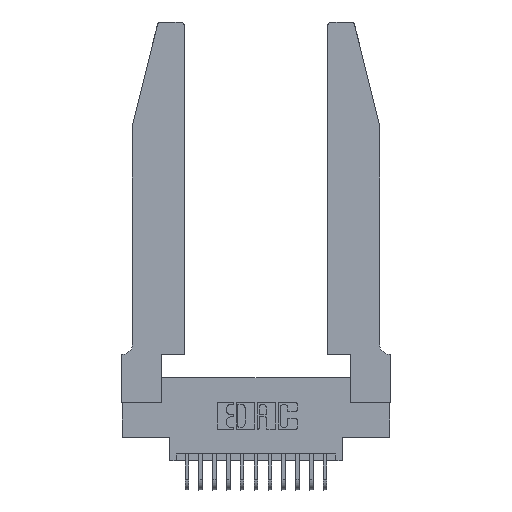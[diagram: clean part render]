
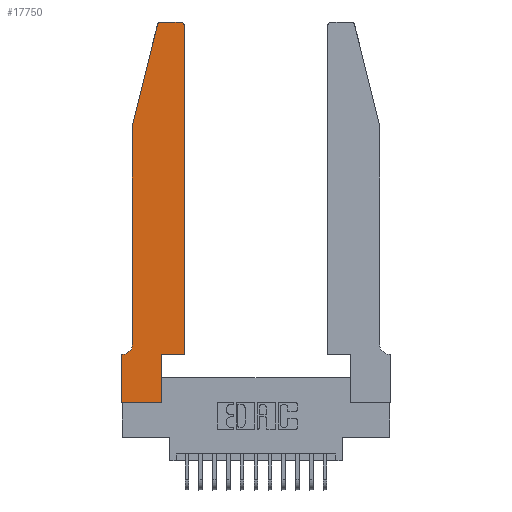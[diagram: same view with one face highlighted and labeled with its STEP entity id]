
A CAD part, top view. The second image highlights one B-rep face of the part: STEP entity #17750.
In plain terms, the highlighted planar face has unit normal (0, 0, 1).
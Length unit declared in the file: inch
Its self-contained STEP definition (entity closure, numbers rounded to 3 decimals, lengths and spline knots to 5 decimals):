
#214 = EDGE_CURVE ( 'NONE', #11306, #16267, #1139, .T. ) ;
#298 = DIRECTION ( 'NONE',  ( -1., 0., 0. ) ) ;
#438 = DIRECTION ( 'NONE',  ( 1., 0., 0. ) ) ;
#689 = AXIS2_PLACEMENT_3D ( 'NONE', #11157, #15512, #16883 ) ;
#804 = ORIENTED_EDGE ( 'NONE', *, *, #7151, .T. ) ;
#845 = ORIENTED_EDGE ( 'NONE', *, *, #3106, .T. ) ;
#929 = CARTESIAN_POINT ( 'NONE',  ( 0.4205, 2.72, 0.37 ) ) ;
#1097 = CARTESIAN_POINT ( 'NONE',  ( 0.0055, 0.35, 0.37 ) ) ;
#1134 = VECTOR ( 'NONE', #3983, 39.37008 ) ;
#1139 = LINE ( 'NONE', #12111, #13782 ) ;
#1180 = DIRECTION ( 'NONE',  ( 0., -1., 0. ) ) ;
#1259 = VERTEX_POINT ( 'NONE', #16466 ) ;
#1511 = VERTEX_POINT ( 'NONE', #18395 ) ;
#1604 = DIRECTION ( 'NONE',  ( 0., 1., 0. ) ) ;
#1765 = VERTEX_POINT ( 'NONE', #13237 ) ;
#1793 = DIRECTION ( 'NONE',  ( -1., 0., 0. ) ) ;
#1834 = EDGE_CURVE ( 'NONE', #12847, #3336, #16252, .T. ) ;
#2216 = LINE ( 'NONE', #17398, #12274 ) ;
#2345 = CARTESIAN_POINT ( 'NONE',  ( 0.0755, 0.35, 0.37 ) ) ;
#2641 = ORIENTED_EDGE ( 'NONE', *, *, #6393, .T. ) ;
#3106 = EDGE_CURVE ( 'NONE', #5735, #12847, #17629, .T. ) ;
#3282 = VERTEX_POINT ( 'NONE', #12560 ) ;
#3287 = VECTOR ( 'NONE', #438, 39.37008 ) ;
#3297 = CARTESIAN_POINT ( 'NONE',  ( 0.2865, 0., 0.37 ) ) ;
#3336 = VERTEX_POINT ( 'NONE', #1097 ) ;
#3373 = ORIENTED_EDGE ( 'NONE', *, *, #16294, .T. ) ;
#3421 = DIRECTION ( 'NONE',  ( 1., 0., 0. ) ) ;
#3604 = ORIENTED_EDGE ( 'NONE', *, *, #1834, .T. ) ;
#3788 = CARTESIAN_POINT ( 'NONE',  ( 0., 0., 0.37 ) ) ;
#3844 = VECTOR ( 'NONE', #7326, 39.37008 ) ;
#3961 = DIRECTION ( 'NONE',  ( 1., 0., 0. ) ) ;
#3983 = DIRECTION ( 'NONE',  ( -1., 0., 0. ) ) ;
#4712 = CARTESIAN_POINT ( 'NONE',  ( 0., 0.35, 0.37 ) ) ;
#5204 = AXIS2_PLACEMENT_3D ( 'NONE', #929, #5391, #3961 ) ;
#5363 = ORIENTED_EDGE ( 'NONE', *, *, #14407, .T. ) ;
#5391 = DIRECTION ( 'NONE',  ( 0., 0., 1. ) ) ;
#5583 = DIRECTION ( 'NONE',  ( -0.239, -0.971, 0. ) ) ;
#5711 = CARTESIAN_POINT ( 'NONE',  ( 0.0755, 0.42, 0.37 ) ) ;
#5735 = VERTEX_POINT ( 'NONE', #15242 ) ;
#6230 = PLANE ( 'NONE',  #6342 ) ;
#6342 = AXIS2_PLACEMENT_3D ( 'NONE', #4712, #7707, #3421 ) ;
#6393 = EDGE_CURVE ( 'NONE', #15076, #12180, #7017, .T. ) ;
#6853 = EDGE_CURVE ( 'NONE', #3282, #1259, #17033, .T. ) ;
#6996 = LINE ( 'NONE', #2345, #1134 ) ;
#7017 = LINE ( 'NONE', #12567, #3287 ) ;
#7028 = EDGE_CURVE ( 'NONE', #1259, #1511, #18914, .T. ) ;
#7151 = EDGE_CURVE ( 'NONE', #10709, #15076, #17489, .T. ) ;
#7326 = DIRECTION ( 'NONE',  ( 0., 1., 0. ) ) ;
#7532 = VECTOR ( 'NONE', #1604, 39.37008 ) ;
#7707 = DIRECTION ( 'NONE',  ( 0., 0., 1. ) ) ;
#9122 = CARTESIAN_POINT ( 'NONE',  ( 0.2865, 0.35, 0.37 ) ) ;
#9790 = VECTOR ( 'NONE', #17410, 39.37008 ) ;
#10137 = ORIENTED_EDGE ( 'NONE', *, *, #19091, .T. ) ;
#10580 = CARTESIAN_POINT ( 'NONE',  ( 0., 0., 0.37 ) ) ;
#10596 = LINE ( 'NONE', #19210, #3844 ) ;
#10644 = VECTOR ( 'NONE', #1180, 39.37008 ) ;
#10709 = VERTEX_POINT ( 'NONE', #11297 ) ;
#10827 = ORIENTED_EDGE ( 'NONE', *, *, #7028, .T. ) ;
#10984 = EDGE_CURVE ( 'NONE', #1511, #5735, #2216, .T. ) ;
#11157 = CARTESIAN_POINT ( 'NONE',  ( 0.284, 2.72, 0.37 ) ) ;
#11297 = CARTESIAN_POINT ( 'NONE',  ( 0., 0.35, 0.37 ) ) ;
#11306 = VERTEX_POINT ( 'NONE', #17693 ) ;
#11874 = CIRCLE ( 'NONE', #5204, 0.03 ) ;
#12111 = CARTESIAN_POINT ( 'NONE',  ( 0.4505, 0.35, 0.37 ) ) ;
#12179 = ORIENTED_EDGE ( 'NONE', *, *, #10984, .T. ) ;
#12180 = VERTEX_POINT ( 'NONE', #3297 ) ;
#12274 = VECTOR ( 'NONE', #5583, 39.37008 ) ;
#12286 = FACE_OUTER_BOUND ( 'NONE', #13163, .T. ) ;
#12386 = VECTOR ( 'NONE', #298, 39.37008 ) ;
#12560 = CARTESIAN_POINT ( 'NONE',  ( 0.4205, 2.75, 0.37 ) ) ;
#12567 = CARTESIAN_POINT ( 'NONE',  ( 0., 0., 0.37 ) ) ;
#12697 = AXIS2_PLACEMENT_3D ( 'NONE', #15348, #16790, #1793 ) ;
#12699 = LINE ( 'NONE', #9122, #7532 ) ;
#12847 = VERTEX_POINT ( 'NONE', #5711 ) ;
#13163 = EDGE_LOOP ( 'NONE', ( #15522, #10827, #12179, #845, #3604, #5363, #804, #2641, #10137, #14003, #18154, #3373 ) ) ;
#13237 = CARTESIAN_POINT ( 'NONE',  ( 0.4505, 2.72, 0.37 ) ) ;
#13782 = VECTOR ( 'NONE', #15254, 39.37008 ) ;
#14003 = ORIENTED_EDGE ( 'NONE', *, *, #214, .T. ) ;
#14390 = CARTESIAN_POINT ( 'NONE',  ( 0.0755, 2., 0.37 ) ) ;
#14407 = EDGE_CURVE ( 'NONE', #3336, #10709, #6996, .T. ) ;
#15076 = VERTEX_POINT ( 'NONE', #10580 ) ;
#15242 = CARTESIAN_POINT ( 'NONE',  ( 0.0755, 2., 0.37 ) ) ;
#15254 = DIRECTION ( 'NONE',  ( 1., 0., 0. ) ) ;
#15348 = CARTESIAN_POINT ( 'NONE',  ( 0.0055, 0.42, 0.37 ) ) ;
#15512 = DIRECTION ( 'NONE',  ( 0., 0., 1. ) ) ;
#15522 = ORIENTED_EDGE ( 'NONE', *, *, #6853, .T. ) ;
#16252 = CIRCLE ( 'NONE', #12697, 0.07 ) ;
#16267 = VERTEX_POINT ( 'NONE', #18850 ) ;
#16290 = CARTESIAN_POINT ( 'NONE',  ( 0.2605, 2.75, 0.37 ) ) ;
#16294 = EDGE_CURVE ( 'NONE', #1765, #3282, #11874, .T. ) ;
#16466 = CARTESIAN_POINT ( 'NONE',  ( 0.284, 2.75, 0.37 ) ) ;
#16790 = DIRECTION ( 'NONE',  ( 0., 0., -1. ) ) ;
#16883 = DIRECTION ( 'NONE',  ( 1., 0., 0. ) ) ;
#17033 = LINE ( 'NONE', #16290, #12386 ) ;
#17398 = CARTESIAN_POINT ( 'NONE',  ( 0.0755, 2., 0.37 ) ) ;
#17410 = DIRECTION ( 'NONE',  ( 0., -1., 0. ) ) ;
#17489 = LINE ( 'NONE', #3788, #9790 ) ;
#17629 = LINE ( 'NONE', #14390, #10644 ) ;
#17693 = CARTESIAN_POINT ( 'NONE',  ( 0.2865, 0.35, 0.37 ) ) ;
#17750 = ADVANCED_FACE ( 'NONE', ( #12286 ), #6230, .T. ) ;
#18154 = ORIENTED_EDGE ( 'NONE', *, *, #18363, .T. ) ;
#18363 = EDGE_CURVE ( 'NONE', #16267, #1765, #10596, .T. ) ;
#18395 = CARTESIAN_POINT ( 'NONE',  ( 0.25487, 2.72718, 0.37 ) ) ;
#18850 = CARTESIAN_POINT ( 'NONE',  ( 0.4505, 0.35, 0.37 ) ) ;
#18914 = CIRCLE ( 'NONE', #689, 0.03 ) ;
#19091 = EDGE_CURVE ( 'NONE', #12180, #11306, #12699, .T. ) ;
#19210 = CARTESIAN_POINT ( 'NONE',  ( 0.4505, 0.35, 0.37 ) ) ;
